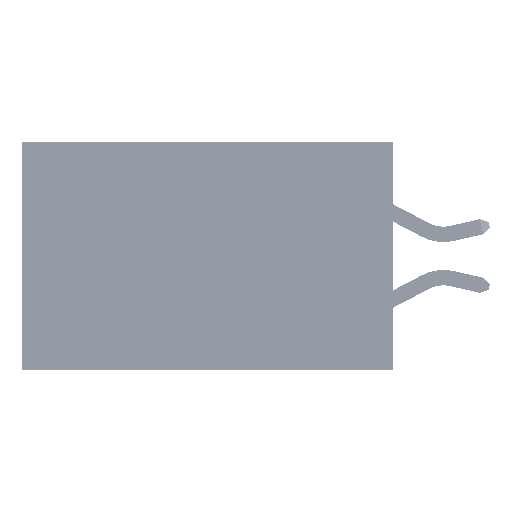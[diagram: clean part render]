
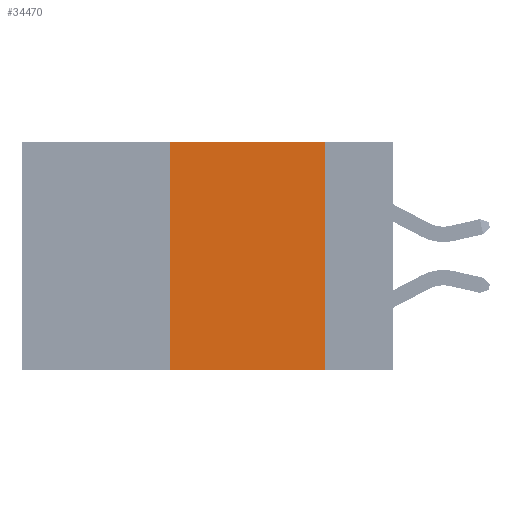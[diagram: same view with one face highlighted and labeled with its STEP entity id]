
A CAD part, left-side view. The second image highlights one B-rep face of the part: STEP entity #34470.
In plain terms, the highlighted planar face has unit normal (-1, 0, 0).
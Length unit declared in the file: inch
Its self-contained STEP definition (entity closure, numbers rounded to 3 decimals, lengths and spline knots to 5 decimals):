
#1782 = VECTOR ( 'NONE', #33194, 39.37008 ) ;
#1931 = DIRECTION ( 'NONE',  ( 0., 0., -1. ) ) ;
#3070 = ORIENTED_EDGE ( 'NONE', *, *, #45960, .T. ) ;
#3144 = CARTESIAN_POINT ( 'NONE',  ( 0., 0.6, -0.37 ) ) ;
#3739 = CARTESIAN_POINT ( 'NONE',  ( 0., 0.6, 0. ) ) ;
#5342 = ORIENTED_EDGE ( 'NONE', *, *, #14733, .F. ) ;
#6150 = EDGE_LOOP ( 'NONE', ( #24035, #5342, #16544, #3070 ) ) ;
#6712 = VECTOR ( 'NONE', #26115, 39.37008 ) ;
#11499 = CARTESIAN_POINT ( 'NONE',  ( 0., 0.36, 0. ) ) ;
#11534 = LINE ( 'NONE', #16860, #29018 ) ;
#11991 = VECTOR ( 'NONE', #33798, 39.37008 ) ;
#13404 = CARTESIAN_POINT ( 'NONE',  ( 0., 0.6, 0. ) ) ;
#14733 = EDGE_CURVE ( 'NONE', #36608, #24155, #26545, .T. ) ;
#14897 = CARTESIAN_POINT ( 'NONE',  ( 0., 0.11, -0.37 ) ) ;
#15409 = CARTESIAN_POINT ( 'NONE',  ( 0., 0.36, -0.37 ) ) ;
#16544 = ORIENTED_EDGE ( 'NONE', *, *, #17744, .F. ) ;
#16860 = CARTESIAN_POINT ( 'NONE',  ( 0., 0.11, 0. ) ) ;
#17744 = EDGE_CURVE ( 'NONE', #37712, #36608, #41571, .T. ) ;
#20848 = DIRECTION ( 'NONE',  ( 0., 0., -1. ) ) ;
#21731 = LINE ( 'NONE', #3144, #1782 ) ;
#24035 = ORIENTED_EDGE ( 'NONE', *, *, #30228, .F. ) ;
#24155 = VERTEX_POINT ( 'NONE', #47720 ) ;
#26115 = DIRECTION ( 'NONE',  ( 0., -1., 0. ) ) ;
#26545 = LINE ( 'NONE', #3739, #6712 ) ;
#29018 = VECTOR ( 'NONE', #1931, 39.37008 ) ;
#30228 = EDGE_CURVE ( 'NONE', #24155, #40785, #11534, .T. ) ;
#30801 = AXIS2_PLACEMENT_3D ( 'NONE', #13404, #43029, #20848 ) ;
#30963 = CARTESIAN_POINT ( 'NONE',  ( 0., 0.36, 0. ) ) ;
#33194 = DIRECTION ( 'NONE',  ( 0., -1., 0. ) ) ;
#33798 = DIRECTION ( 'NONE',  ( 0., 0., 1. ) ) ;
#34470 = ADVANCED_FACE ( 'NONE', ( #43251 ), #35627, .F. ) ;
#35627 = PLANE ( 'NONE',  #30801 ) ;
#36608 = VERTEX_POINT ( 'NONE', #30963 ) ;
#37712 = VERTEX_POINT ( 'NONE', #15409 ) ;
#40785 = VERTEX_POINT ( 'NONE', #14897 ) ;
#41571 = LINE ( 'NONE', #11499, #11991 ) ;
#43029 = DIRECTION ( 'NONE',  ( 1., 0., 0. ) ) ;
#43251 = FACE_OUTER_BOUND ( 'NONE', #6150, .T. ) ;
#45960 = EDGE_CURVE ( 'NONE', #37712, #40785, #21731, .T. ) ;
#47720 = CARTESIAN_POINT ( 'NONE',  ( 0., 0.11, 0. ) ) ;
